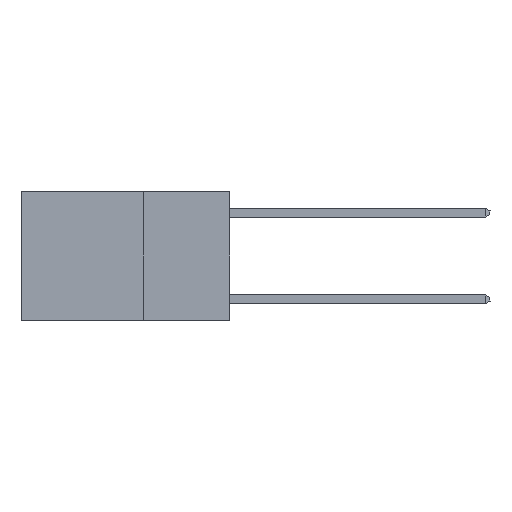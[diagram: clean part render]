
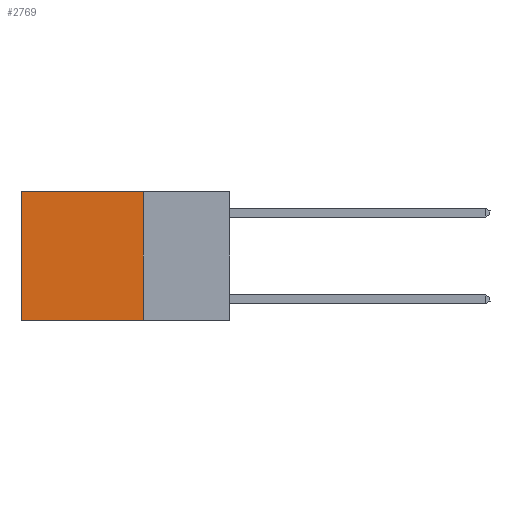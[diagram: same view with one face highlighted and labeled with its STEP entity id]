
A CAD part, left-side view. The second image highlights one B-rep face of the part: STEP entity #2769.
In plain terms, the highlighted planar face has unit normal (-1, 0, 0).
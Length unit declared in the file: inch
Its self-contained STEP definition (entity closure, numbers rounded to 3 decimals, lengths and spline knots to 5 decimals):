
#150 = AXIS2_PLACEMENT_3D ( 'NONE', #14857, #2986, #1538 ) ;
#249 = LINE ( 'NONE', #1759, #1673 ) ;
#853 = VERTEX_POINT ( 'NONE', #14793 ) ;
#1538 = DIRECTION ( 'NONE',  ( 0., 0., -1. ) ) ;
#1660 = VECTOR ( 'NONE', #15210, 39.37008 ) ;
#1673 = VECTOR ( 'NONE', #15077, 39.37008 ) ;
#1759 = CARTESIAN_POINT ( 'NONE',  ( 0.2625, 0.25, -0.37 ) ) ;
#1979 = LINE ( 'NONE', #5791, #1660 ) ;
#2153 = VERTEX_POINT ( 'NONE', #10621 ) ;
#2193 = VECTOR ( 'NONE', #9581, 39.37008 ) ;
#2655 = LINE ( 'NONE', #17435, #11252 ) ;
#2769 = ADVANCED_FACE ( 'NONE', ( #16381 ), #13614, .F. ) ;
#2986 = DIRECTION ( 'NONE',  ( 1., 0., 0. ) ) ;
#3594 = ORIENTED_EDGE ( 'NONE', *, *, #5644, .F. ) ;
#3740 = CARTESIAN_POINT ( 'NONE',  ( 0.2625, 0.25, -0.37 ) ) ;
#3807 = VERTEX_POINT ( 'NONE', #9990 ) ;
#4460 = EDGE_CURVE ( 'NONE', #3807, #8493, #2655, .T. ) ;
#4646 = ORIENTED_EDGE ( 'NONE', *, *, #5273, .T. ) ;
#5273 = EDGE_CURVE ( 'NONE', #853, #2153, #1979, .T. ) ;
#5644 = EDGE_CURVE ( 'NONE', #8493, #2153, #249, .T. ) ;
#5791 = CARTESIAN_POINT ( 'NONE',  ( 0.2625, 0.6, 0. ) ) ;
#6678 = ORIENTED_EDGE ( 'NONE', *, *, #4460, .F. ) ;
#6770 = LINE ( 'NONE', #17464, #2193 ) ;
#8493 = VERTEX_POINT ( 'NONE', #3740 ) ;
#9031 = DIRECTION ( 'NONE',  ( 0., 0., -1. ) ) ;
#9581 = DIRECTION ( 'NONE',  ( 0., 1., 0. ) ) ;
#9990 = CARTESIAN_POINT ( 'NONE',  ( 0.2625, 0.25, 0. ) ) ;
#10621 = CARTESIAN_POINT ( 'NONE',  ( 0.2625, 0.6, -0.37 ) ) ;
#11252 = VECTOR ( 'NONE', #9031, 39.37008 ) ;
#13614 = PLANE ( 'NONE',  #150 ) ;
#14013 = EDGE_LOOP ( 'NONE', ( #4646, #3594, #6678, #14547 ) ) ;
#14547 = ORIENTED_EDGE ( 'NONE', *, *, #14738, .T. ) ;
#14738 = EDGE_CURVE ( 'NONE', #3807, #853, #6770, .T. ) ;
#14793 = CARTESIAN_POINT ( 'NONE',  ( 0.2625, 0.6, 0. ) ) ;
#14857 = CARTESIAN_POINT ( 'NONE',  ( 0.2625, 0.25, 0. ) ) ;
#15077 = DIRECTION ( 'NONE',  ( 0., 1., 0. ) ) ;
#15210 = DIRECTION ( 'NONE',  ( 0., 0., -1. ) ) ;
#16381 = FACE_OUTER_BOUND ( 'NONE', #14013, .T. ) ;
#17435 = CARTESIAN_POINT ( 'NONE',  ( 0.2625, 0.25, 0. ) ) ;
#17464 = CARTESIAN_POINT ( 'NONE',  ( 0.2625, 0.25, 0. ) ) ;
